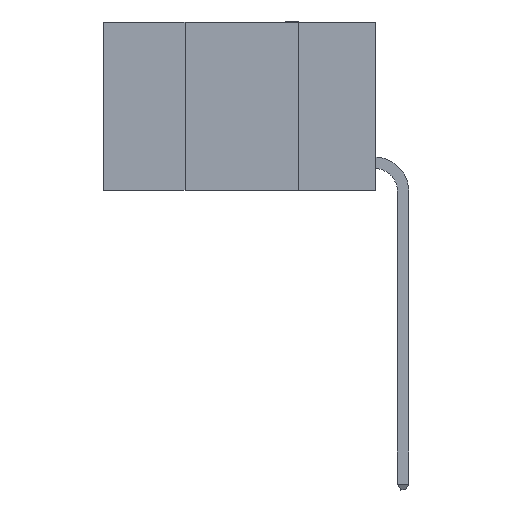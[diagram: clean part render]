
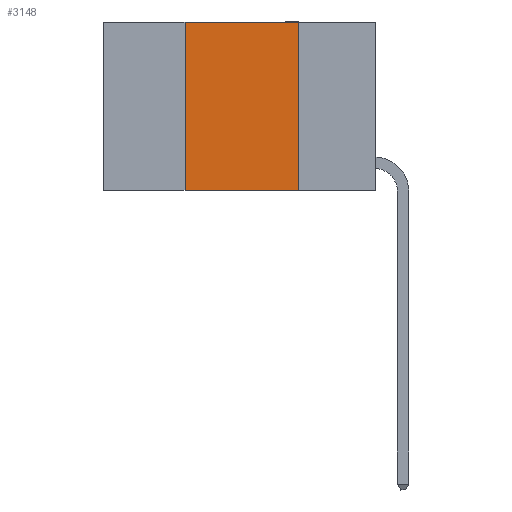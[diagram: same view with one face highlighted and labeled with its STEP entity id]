
A CAD part, left-side view. The second image highlights one B-rep face of the part: STEP entity #3148.
In plain terms, the highlighted planar face has unit normal (-1, 0, 0).
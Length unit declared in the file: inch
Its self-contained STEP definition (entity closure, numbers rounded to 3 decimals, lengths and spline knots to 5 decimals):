
#1711 = CARTESIAN_POINT ( 'NONE',  ( 0., 0.17, -0.37 ) ) ;
#2439 = DIRECTION ( 'NONE',  ( 1., 0., 0. ) ) ;
#2901 = VERTEX_POINT ( 'NONE', #1711 ) ;
#3148 = ADVANCED_FACE ( 'NONE', ( #11360 ), #14149, .F. ) ;
#3919 = LINE ( 'NONE', #15818, #9397 ) ;
#4242 = CARTESIAN_POINT ( 'NONE',  ( 0., 0.6, -0.37 ) ) ;
#4634 = ORIENTED_EDGE ( 'NONE', *, *, #14826, .F. ) ;
#5511 = VECTOR ( 'NONE', #5659, 39.37008 ) ;
#5659 = DIRECTION ( 'NONE',  ( 0., -1., 0. ) ) ;
#5778 = VERTEX_POINT ( 'NONE', #12955 ) ;
#6124 = DIRECTION ( 'NONE',  ( 0., 0., 1. ) ) ;
#6207 = EDGE_CURVE ( 'NONE', #8882, #2901, #3919, .T. ) ;
#6337 = DIRECTION ( 'NONE',  ( 0., 0., -1. ) ) ;
#6686 = CARTESIAN_POINT ( 'NONE',  ( 0., 0.17, 0. ) ) ;
#8459 = EDGE_CURVE ( 'NONE', #5778, #2901, #13154, .T. ) ;
#8783 = AXIS2_PLACEMENT_3D ( 'NONE', #13984, #2439, #6337 ) ;
#8882 = VERTEX_POINT ( 'NONE', #6686 ) ;
#9397 = VECTOR ( 'NONE', #11998, 39.37008 ) ;
#9616 = EDGE_CURVE ( 'NONE', #5778, #12233, #12500, .T. ) ;
#11075 = VECTOR ( 'NONE', #15792, 39.37008 ) ;
#11277 = ORIENTED_EDGE ( 'NONE', *, *, #9616, .F. ) ;
#11360 = FACE_OUTER_BOUND ( 'NONE', #15904, .T. ) ;
#11998 = DIRECTION ( 'NONE',  ( 0., 0., -1. ) ) ;
#12233 = VERTEX_POINT ( 'NONE', #13387 ) ;
#12500 = LINE ( 'NONE', #12745, #16223 ) ;
#12745 = CARTESIAN_POINT ( 'NONE',  ( 0., 0.42, 0. ) ) ;
#12955 = CARTESIAN_POINT ( 'NONE',  ( 0., 0.42, -0.37 ) ) ;
#13040 = ORIENTED_EDGE ( 'NONE', *, *, #8459, .T. ) ;
#13154 = LINE ( 'NONE', #4242, #11075 ) ;
#13305 = LINE ( 'NONE', #14663, #5511 ) ;
#13387 = CARTESIAN_POINT ( 'NONE',  ( 0., 0.42, 0. ) ) ;
#13984 = CARTESIAN_POINT ( 'NONE',  ( 0., 0.6, 0. ) ) ;
#14149 = PLANE ( 'NONE',  #8783 ) ;
#14161 = ORIENTED_EDGE ( 'NONE', *, *, #6207, .F. ) ;
#14663 = CARTESIAN_POINT ( 'NONE',  ( 0., 0.6, 0. ) ) ;
#14826 = EDGE_CURVE ( 'NONE', #12233, #8882, #13305, .T. ) ;
#15792 = DIRECTION ( 'NONE',  ( 0., -1., 0. ) ) ;
#15818 = CARTESIAN_POINT ( 'NONE',  ( 0., 0.17, 0. ) ) ;
#15904 = EDGE_LOOP ( 'NONE', ( #14161, #4634, #11277, #13040 ) ) ;
#16223 = VECTOR ( 'NONE', #6124, 39.37008 ) ;
